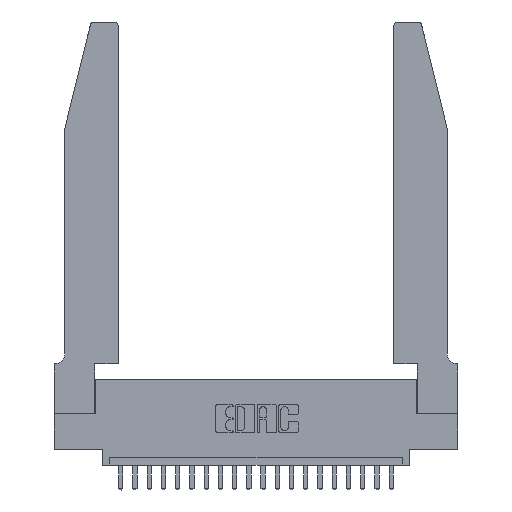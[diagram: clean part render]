
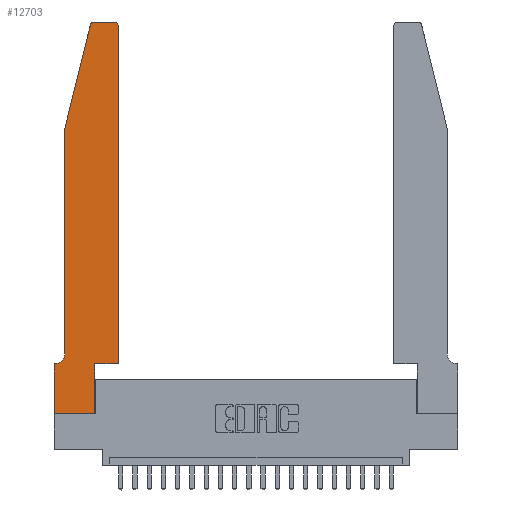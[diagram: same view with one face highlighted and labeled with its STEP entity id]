
A CAD part, top view. The second image highlights one B-rep face of the part: STEP entity #12703.
In plain terms, the highlighted planar face has unit normal (0, 0, 1).
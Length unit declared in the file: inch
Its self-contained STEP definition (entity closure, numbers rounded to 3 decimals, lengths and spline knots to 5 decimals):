
#209 = ORIENTED_EDGE ( 'NONE', *, *, #8699, .T. ) ;
#306 = ORIENTED_EDGE ( 'NONE', *, *, #16747, .T. ) ;
#350 = VERTEX_POINT ( 'NONE', #1819 ) ;
#976 = LINE ( 'NONE', #13641, #1797 ) ;
#1406 = ORIENTED_EDGE ( 'NONE', *, *, #21045, .T. ) ;
#1797 = VECTOR ( 'NONE', #22444, 39.37008 ) ;
#1819 = CARTESIAN_POINT ( 'NONE',  ( 0.2865, 0., 0.37 ) ) ;
#1832 = VERTEX_POINT ( 'NONE', #17797 ) ;
#2030 = CARTESIAN_POINT ( 'NONE',  ( 0., 0., 0.37 ) ) ;
#2228 = DIRECTION ( 'NONE',  ( 1., 0., 0. ) ) ;
#2314 = LINE ( 'NONE', #10808, #20628 ) ;
#2360 = VERTEX_POINT ( 'NONE', #12756 ) ;
#2444 = ORIENTED_EDGE ( 'NONE', *, *, #22268, .T. ) ;
#2679 = CARTESIAN_POINT ( 'NONE',  ( 0.4505, 0.35, 0.37 ) ) ;
#2720 = DIRECTION ( 'NONE',  ( 0., 0., 1. ) ) ;
#3166 = CARTESIAN_POINT ( 'NONE',  ( 0.4205, 2.72, 0.37 ) ) ;
#3447 = VERTEX_POINT ( 'NONE', #22372 ) ;
#3491 = LINE ( 'NONE', #14289, #6032 ) ;
#3626 = CARTESIAN_POINT ( 'NONE',  ( 0.0755, 2., 0.37 ) ) ;
#3645 = ORIENTED_EDGE ( 'NONE', *, *, #21806, .T. ) ;
#4215 = LINE ( 'NONE', #2679, #12838 ) ;
#4339 = VERTEX_POINT ( 'NONE', #19998 ) ;
#4370 = LINE ( 'NONE', #22933, #14904 ) ;
#4605 = ORIENTED_EDGE ( 'NONE', *, *, #13445, .T. ) ;
#4947 = CIRCLE ( 'NONE', #19927, 0.03 ) ;
#5436 = DIRECTION ( 'NONE',  ( 0., 0., 1. ) ) ;
#5547 = DIRECTION ( 'NONE',  ( 0., -1., 0. ) ) ;
#5595 = CARTESIAN_POINT ( 'NONE',  ( 0.284, 2.72, 0.37 ) ) ;
#6032 = VECTOR ( 'NONE', #8958, 39.37008 ) ;
#6105 = CIRCLE ( 'NONE', #17958, 0.03 ) ;
#6576 = VECTOR ( 'NONE', #15727, 39.37008 ) ;
#6926 = ORIENTED_EDGE ( 'NONE', *, *, #22473, .T. ) ;
#7145 = EDGE_CURVE ( 'NONE', #11514, #4339, #14851, .T. ) ;
#7259 = VERTEX_POINT ( 'NONE', #11551 ) ;
#7596 = CARTESIAN_POINT ( 'NONE',  ( 0.0755, 2., 0.37 ) ) ;
#7678 = DIRECTION ( 'NONE',  ( 0., -1., 0. ) ) ;
#8228 = LINE ( 'NONE', #10282, #6576 ) ;
#8699 = EDGE_CURVE ( 'NONE', #13969, #21760, #21210, .T. ) ;
#8794 = DIRECTION ( 'NONE',  ( 1., 0., 0. ) ) ;
#8958 = DIRECTION ( 'NONE',  ( -1., 0., 0. ) ) ;
#10133 = PLANE ( 'NONE',  #12851 ) ;
#10263 = CARTESIAN_POINT ( 'NONE',  ( 0.0055, 0.35, 0.37 ) ) ;
#10282 = CARTESIAN_POINT ( 'NONE',  ( 0.0755, 0.35, 0.37 ) ) ;
#10431 = EDGE_LOOP ( 'NONE', ( #6926, #3645, #18623, #209, #1406, #4605, #17511, #2444, #14022, #11736, #306, #21269 ) ) ;
#10465 = VECTOR ( 'NONE', #2228, 39.37008 ) ;
#10648 = CARTESIAN_POINT ( 'NONE',  ( 0.0055, 0.42, 0.37 ) ) ;
#10722 = CARTESIAN_POINT ( 'NONE',  ( 0.0755, 0.42, 0.37 ) ) ;
#10808 = CARTESIAN_POINT ( 'NONE',  ( 0.2865, 0.35, 0.37 ) ) ;
#11514 = VERTEX_POINT ( 'NONE', #11647 ) ;
#11551 = CARTESIAN_POINT ( 'NONE',  ( 0., 0.35, 0.37 ) ) ;
#11647 = CARTESIAN_POINT ( 'NONE',  ( 0.2865, 0.35, 0.37 ) ) ;
#11736 = ORIENTED_EDGE ( 'NONE', *, *, #7145, .T. ) ;
#11824 = DIRECTION ( 'NONE',  ( 1., 0., 0. ) ) ;
#12056 = CARTESIAN_POINT ( 'NONE',  ( 0.284, 2.75, 0.37 ) ) ;
#12703 = ADVANCED_FACE ( 'NONE', ( #22152 ), #10133, .T. ) ;
#12756 = CARTESIAN_POINT ( 'NONE',  ( 0.4205, 2.75, 0.37 ) ) ;
#12838 = VECTOR ( 'NONE', #22270, 39.37008 ) ;
#12851 = AXIS2_PLACEMENT_3D ( 'NONE', #15438, #2720, #22551 ) ;
#13073 = LINE ( 'NONE', #2030, #13345 ) ;
#13345 = VECTOR ( 'NONE', #5547, 39.37008 ) ;
#13445 = EDGE_CURVE ( 'NONE', #13530, #7259, #8228, .T. ) ;
#13515 = CIRCLE ( 'NONE', #14411, 0.07 ) ;
#13530 = VERTEX_POINT ( 'NONE', #10263 ) ;
#13641 = CARTESIAN_POINT ( 'NONE',  ( 0.0755, 2., 0.37 ) ) ;
#13969 = VERTEX_POINT ( 'NONE', #3626 ) ;
#14022 = ORIENTED_EDGE ( 'NONE', *, *, #15870, .T. ) ;
#14289 = CARTESIAN_POINT ( 'NONE',  ( 0.2605, 2.75, 0.37 ) ) ;
#14411 = AXIS2_PLACEMENT_3D ( 'NONE', #10648, #14641, #19090 ) ;
#14415 = EDGE_CURVE ( 'NONE', #3447, #13969, #976, .T. ) ;
#14641 = DIRECTION ( 'NONE',  ( 0., 0., -1. ) ) ;
#14851 = LINE ( 'NONE', #20225, #10465 ) ;
#14904 = VECTOR ( 'NONE', #8794, 39.37008 ) ;
#15438 = CARTESIAN_POINT ( 'NONE',  ( 0., 0.35, 0.37 ) ) ;
#15550 = CARTESIAN_POINT ( 'NONE',  ( 0.4505, 2.72, 0.37 ) ) ;
#15727 = DIRECTION ( 'NONE',  ( -1., 0., 0. ) ) ;
#15870 = EDGE_CURVE ( 'NONE', #350, #11514, #2314, .T. ) ;
#16269 = DIRECTION ( 'NONE',  ( 0., 1., 0. ) ) ;
#16747 = EDGE_CURVE ( 'NONE', #4339, #18335, #4215, .T. ) ;
#17033 = EDGE_CURVE ( 'NONE', #7259, #1832, #13073, .T. ) ;
#17511 = ORIENTED_EDGE ( 'NONE', *, *, #17033, .T. ) ;
#17597 = VECTOR ( 'NONE', #7678, 39.37008 ) ;
#17797 = CARTESIAN_POINT ( 'NONE',  ( 0., 0., 0.37 ) ) ;
#17958 = AXIS2_PLACEMENT_3D ( 'NONE', #3166, #22628, #11824 ) ;
#18187 = EDGE_CURVE ( 'NONE', #18335, #2360, #6105, .T. ) ;
#18335 = VERTEX_POINT ( 'NONE', #15550 ) ;
#18623 = ORIENTED_EDGE ( 'NONE', *, *, #14415, .T. ) ;
#19090 = DIRECTION ( 'NONE',  ( -1., 0., 0. ) ) ;
#19843 = DIRECTION ( 'NONE',  ( 1., 0., 0. ) ) ;
#19927 = AXIS2_PLACEMENT_3D ( 'NONE', #5595, #5436, #19843 ) ;
#19998 = CARTESIAN_POINT ( 'NONE',  ( 0.4505, 0.35, 0.37 ) ) ;
#20225 = CARTESIAN_POINT ( 'NONE',  ( 0.4505, 0.35, 0.37 ) ) ;
#20577 = VERTEX_POINT ( 'NONE', #12056 ) ;
#20628 = VECTOR ( 'NONE', #16269, 39.37008 ) ;
#21045 = EDGE_CURVE ( 'NONE', #21760, #13530, #13515, .T. ) ;
#21210 = LINE ( 'NONE', #7596, #17597 ) ;
#21269 = ORIENTED_EDGE ( 'NONE', *, *, #18187, .T. ) ;
#21760 = VERTEX_POINT ( 'NONE', #10722 ) ;
#21806 = EDGE_CURVE ( 'NONE', #20577, #3447, #4947, .T. ) ;
#22152 = FACE_OUTER_BOUND ( 'NONE', #10431, .T. ) ;
#22268 = EDGE_CURVE ( 'NONE', #1832, #350, #4370, .T. ) ;
#22270 = DIRECTION ( 'NONE',  ( 0., 1., 0. ) ) ;
#22372 = CARTESIAN_POINT ( 'NONE',  ( 0.25487, 2.72718, 0.37 ) ) ;
#22444 = DIRECTION ( 'NONE',  ( -0.239, -0.971, 0. ) ) ;
#22473 = EDGE_CURVE ( 'NONE', #2360, #20577, #3491, .T. ) ;
#22551 = DIRECTION ( 'NONE',  ( 1., 0., 0. ) ) ;
#22628 = DIRECTION ( 'NONE',  ( 0., 0., 1. ) ) ;
#22933 = CARTESIAN_POINT ( 'NONE',  ( 0., 0., 0.37 ) ) ;
